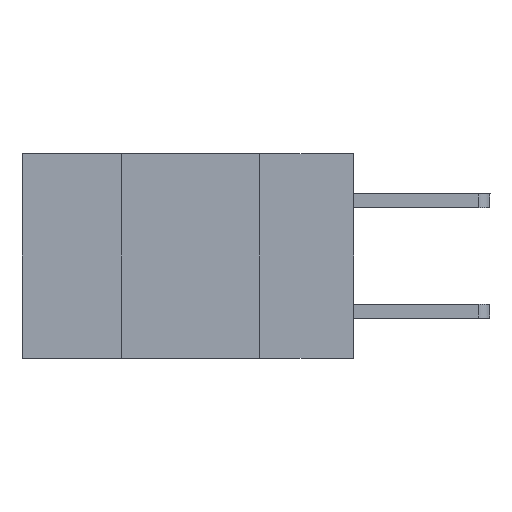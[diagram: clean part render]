
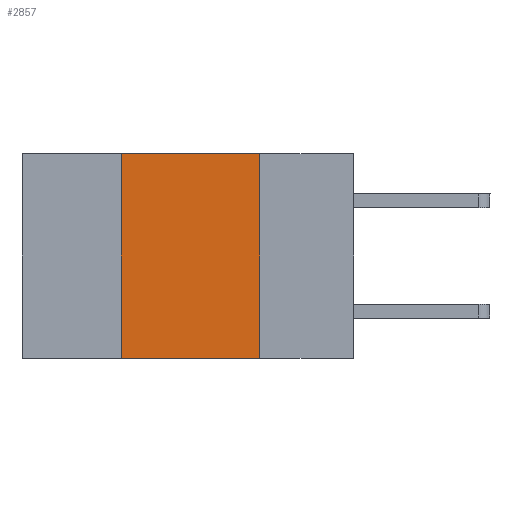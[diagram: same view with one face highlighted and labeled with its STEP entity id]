
A CAD part, left-side view. The second image highlights one B-rep face of the part: STEP entity #2857.
In plain terms, the highlighted planar face has unit normal (-1, 0, 0).
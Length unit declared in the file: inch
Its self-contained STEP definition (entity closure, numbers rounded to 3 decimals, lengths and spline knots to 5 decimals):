
#109 = CARTESIAN_POINT ( 'NONE',  ( 0., 0.42, -0.37 ) ) ;
#216 = ORIENTED_EDGE ( 'NONE', *, *, #9128, .F. ) ;
#235 = VERTEX_POINT ( 'NONE', #4372 ) ;
#285 = ORIENTED_EDGE ( 'NONE', *, *, #6936, .F. ) ;
#571 = DIRECTION ( 'NONE',  ( 1., 0., 0. ) ) ;
#781 = LINE ( 'NONE', #8768, #3561 ) ;
#841 = VECTOR ( 'NONE', #6367, 39.37008 ) ;
#1185 = CARTESIAN_POINT ( 'NONE',  ( 0., 0.17, 0. ) ) ;
#1456 = CARTESIAN_POINT ( 'NONE',  ( 0., 0.6, 0. ) ) ;
#1706 = ORIENTED_EDGE ( 'NONE', *, *, #4194, .F. ) ;
#2519 = VERTEX_POINT ( 'NONE', #109 ) ;
#2857 = ADVANCED_FACE ( 'NONE', ( #5091 ), #9507, .F. ) ;
#3023 = CARTESIAN_POINT ( 'NONE',  ( 0., 0.17, 0. ) ) ;
#3109 = VECTOR ( 'NONE', #4982, 39.37008 ) ;
#3561 = VECTOR ( 'NONE', #9469, 39.37008 ) ;
#3881 = VERTEX_POINT ( 'NONE', #9373 ) ;
#3961 = EDGE_CURVE ( 'NONE', #2519, #3881, #781, .T. ) ;
#4022 = LINE ( 'NONE', #7947, #3109 ) ;
#4183 = CARTESIAN_POINT ( 'NONE',  ( 0., 0.6, 0. ) ) ;
#4194 = EDGE_CURVE ( 'NONE', #2519, #235, #4022, .T. ) ;
#4252 = VERTEX_POINT ( 'NONE', #3023 ) ;
#4372 = CARTESIAN_POINT ( 'NONE',  ( 0., 0.42, 0. ) ) ;
#4495 = ORIENTED_EDGE ( 'NONE', *, *, #3961, .T. ) ;
#4897 = EDGE_LOOP ( 'NONE', ( #285, #216, #1706, #4495 ) ) ;
#4982 = DIRECTION ( 'NONE',  ( 0., 0., 1. ) ) ;
#5091 = FACE_OUTER_BOUND ( 'NONE', #4897, .T. ) ;
#5092 = AXIS2_PLACEMENT_3D ( 'NONE', #4183, #571, #9374 ) ;
#6044 = LINE ( 'NONE', #1456, #6750 ) ;
#6367 = DIRECTION ( 'NONE',  ( 0., 0., -1. ) ) ;
#6750 = VECTOR ( 'NONE', #7379, 39.37008 ) ;
#6936 = EDGE_CURVE ( 'NONE', #4252, #3881, #8731, .T. ) ;
#7379 = DIRECTION ( 'NONE',  ( 0., -1., 0. ) ) ;
#7947 = CARTESIAN_POINT ( 'NONE',  ( 0., 0.42, 0. ) ) ;
#8731 = LINE ( 'NONE', #1185, #841 ) ;
#8768 = CARTESIAN_POINT ( 'NONE',  ( 0., 0.6, -0.37 ) ) ;
#9128 = EDGE_CURVE ( 'NONE', #235, #4252, #6044, .T. ) ;
#9373 = CARTESIAN_POINT ( 'NONE',  ( 0., 0.17, -0.37 ) ) ;
#9374 = DIRECTION ( 'NONE',  ( 0., 0., -1. ) ) ;
#9469 = DIRECTION ( 'NONE',  ( 0., -1., 0. ) ) ;
#9507 = PLANE ( 'NONE',  #5092 ) ;
